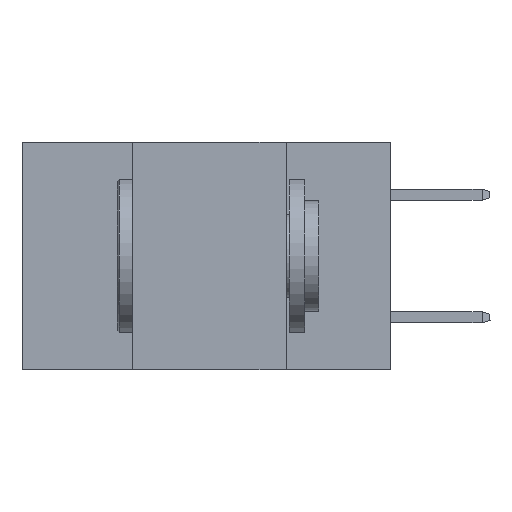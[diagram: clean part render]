
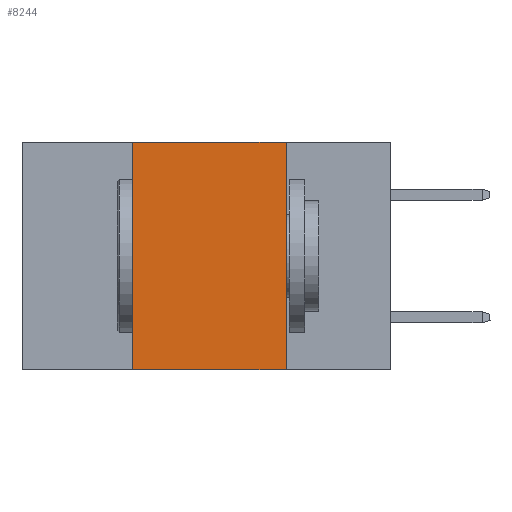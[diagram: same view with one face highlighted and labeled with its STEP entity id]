
A CAD part, left-side view. The second image highlights one B-rep face of the part: STEP entity #8244.
In plain terms, the highlighted planar face has unit normal (-1, 0, 0).
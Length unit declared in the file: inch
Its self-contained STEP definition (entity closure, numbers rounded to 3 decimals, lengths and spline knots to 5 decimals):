
#200 = ORIENTED_EDGE ( 'NONE', *, *, #10843, .F. ) ;
#1785 = CARTESIAN_POINT ( 'NONE',  ( 0., 0.42, -0.37 ) ) ;
#1829 = ORIENTED_EDGE ( 'NONE', *, *, #9881, .T. ) ;
#2627 = VERTEX_POINT ( 'NONE', #15579 ) ;
#2661 = ORIENTED_EDGE ( 'NONE', *, *, #3037, .F. ) ;
#3037 = EDGE_CURVE ( 'NONE', #24747, #15805, #3254, .T. ) ;
#3254 = LINE ( 'NONE', #12931, #12679 ) ;
#3479 = CARTESIAN_POINT ( 'NONE',  ( 0., 0.42, 0. ) ) ;
#3533 = DIRECTION ( 'NONE',  ( 0., -1., 0. ) ) ;
#3651 = DIRECTION ( 'NONE',  ( 0., 0., -1. ) ) ;
#4301 = ORIENTED_EDGE ( 'NONE', *, *, #26310, .F. ) ;
#5742 = CARTESIAN_POINT ( 'NONE',  ( 0., 0.17, 0. ) ) ;
#6179 = LINE ( 'NONE', #7886, #24394 ) ;
#7886 = CARTESIAN_POINT ( 'NONE',  ( 0., 0.17, 0. ) ) ;
#7999 = DIRECTION ( 'NONE',  ( 1., 0., 0. ) ) ;
#8244 = ADVANCED_FACE ( 'NONE', ( #20509 ), #16790, .F. ) ;
#8965 = VERTEX_POINT ( 'NONE', #1785 ) ;
#9881 = EDGE_CURVE ( 'NONE', #8965, #2627, #26490, .T. ) ;
#10063 = CARTESIAN_POINT ( 'NONE',  ( 0., 0.6, 0. ) ) ;
#10843 = EDGE_CURVE ( 'NONE', #15805, #2627, #6179, .T. ) ;
#12533 = EDGE_LOOP ( 'NONE', ( #200, #2661, #4301, #1829 ) ) ;
#12625 = VECTOR ( 'NONE', #3533, 39.37008 ) ;
#12679 = VECTOR ( 'NONE', #17301, 39.37008 ) ;
#12916 = LINE ( 'NONE', #3479, #17018 ) ;
#12927 = AXIS2_PLACEMENT_3D ( 'NONE', #10063, #7999, #3651 ) ;
#12931 = CARTESIAN_POINT ( 'NONE',  ( 0., 0.6, 0. ) ) ;
#15579 = CARTESIAN_POINT ( 'NONE',  ( 0., 0.17, -0.37 ) ) ;
#15805 = VERTEX_POINT ( 'NONE', #5742 ) ;
#16489 = CARTESIAN_POINT ( 'NONE',  ( 0., 0.6, -0.37 ) ) ;
#16498 = DIRECTION ( 'NONE',  ( 0., 0., -1. ) ) ;
#16790 = PLANE ( 'NONE',  #12927 ) ;
#17018 = VECTOR ( 'NONE', #22915, 39.37008 ) ;
#17301 = DIRECTION ( 'NONE',  ( 0., -1., 0. ) ) ;
#20509 = FACE_OUTER_BOUND ( 'NONE', #12533, .T. ) ;
#20548 = CARTESIAN_POINT ( 'NONE',  ( 0., 0.42, 0. ) ) ;
#22915 = DIRECTION ( 'NONE',  ( 0., 0., 1. ) ) ;
#24394 = VECTOR ( 'NONE', #16498, 39.37008 ) ;
#24747 = VERTEX_POINT ( 'NONE', #20548 ) ;
#26310 = EDGE_CURVE ( 'NONE', #8965, #24747, #12916, .T. ) ;
#26490 = LINE ( 'NONE', #16489, #12625 ) ;
